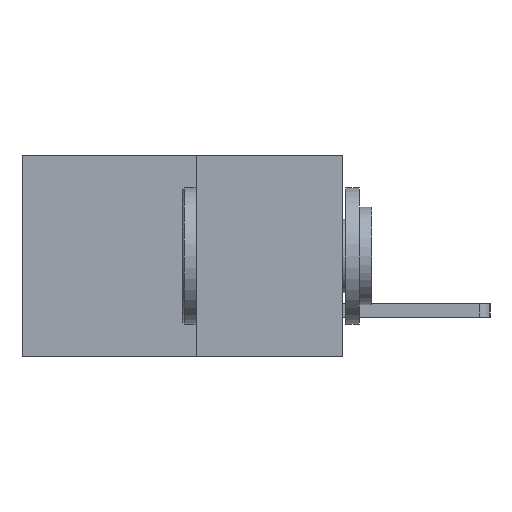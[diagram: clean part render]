
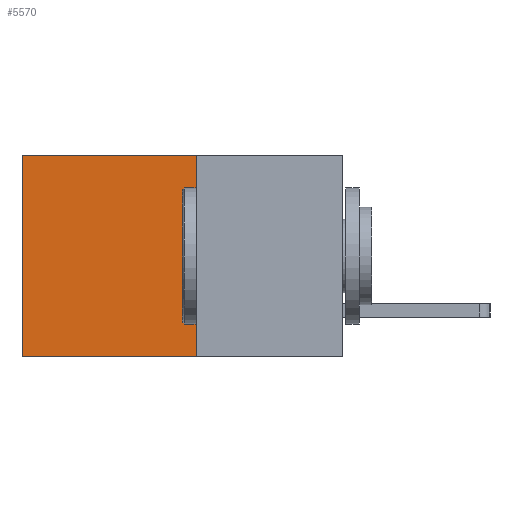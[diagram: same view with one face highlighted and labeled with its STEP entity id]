
A CAD part, left-side view. The second image highlights one B-rep face of the part: STEP entity #5570.
In plain terms, the highlighted planar face has unit normal (-1, 0, 0).
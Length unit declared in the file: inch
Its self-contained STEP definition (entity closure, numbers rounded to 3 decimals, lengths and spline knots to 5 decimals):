
#22 = ORIENTED_EDGE ( 'NONE', *, *, #4713, .T. ) ;
#277 = EDGE_CURVE ( 'NONE', #1090, #2501, #8124, .T. ) ;
#381 = DIRECTION ( 'NONE',  ( 0., 0., -1. ) ) ;
#455 = VECTOR ( 'NONE', #1101, 39.37008 ) ;
#534 = DIRECTION ( 'NONE',  ( 1., 0., 0. ) ) ;
#548 = CARTESIAN_POINT ( 'NONE',  ( 0.277, 0.27, -0.37 ) ) ;
#688 = PLANE ( 'NONE',  #2563 ) ;
#1090 = VERTEX_POINT ( 'NONE', #5606 ) ;
#1101 = DIRECTION ( 'NONE',  ( 0., 0., -1. ) ) ;
#1481 = CARTESIAN_POINT ( 'NONE',  ( 0.277, 0.27, -0.37 ) ) ;
#1509 = EDGE_LOOP ( 'NONE', ( #22, #2766, #8586, #7728 ) ) ;
#2123 = VERTEX_POINT ( 'NONE', #7478 ) ;
#2501 = VERTEX_POINT ( 'NONE', #4566 ) ;
#2563 = AXIS2_PLACEMENT_3D ( 'NONE', #548, #534, #381 ) ;
#2648 = VECTOR ( 'NONE', #8681, 39.37008 ) ;
#2766 = ORIENTED_EDGE ( 'NONE', *, *, #277, .F. ) ;
#4310 = LINE ( 'NONE', #1481, #455 ) ;
#4478 = CARTESIAN_POINT ( 'NONE',  ( 0.277, 0.27, 0. ) ) ;
#4566 = CARTESIAN_POINT ( 'NONE',  ( 0.277, 0.59, -0.37 ) ) ;
#4713 = EDGE_CURVE ( 'NONE', #2123, #2501, #5954, .T. ) ;
#5328 = EDGE_CURVE ( 'NONE', #7830, #2123, #7575, .T. ) ;
#5570 = ADVANCED_FACE ( 'NONE', ( #7466 ), #688, .F. ) ;
#5606 = CARTESIAN_POINT ( 'NONE',  ( 0.277, 0.27, -0.37 ) ) ;
#5683 = VECTOR ( 'NONE', #8881, 39.37008 ) ;
#5719 = VECTOR ( 'NONE', #7019, 39.37008 ) ;
#5932 = CARTESIAN_POINT ( 'NONE',  ( 0.277, 0.27, -0.37 ) ) ;
#5954 = LINE ( 'NONE', #7749, #5719 ) ;
#6415 = EDGE_CURVE ( 'NONE', #7830, #1090, #4310, .T. ) ;
#7019 = DIRECTION ( 'NONE',  ( 0., 0., -1. ) ) ;
#7466 = FACE_OUTER_BOUND ( 'NONE', #1509, .T. ) ;
#7478 = CARTESIAN_POINT ( 'NONE',  ( 0.277, 0.59, 0. ) ) ;
#7575 = LINE ( 'NONE', #8238, #5683 ) ;
#7728 = ORIENTED_EDGE ( 'NONE', *, *, #5328, .T. ) ;
#7749 = CARTESIAN_POINT ( 'NONE',  ( 0.277, 0.59, -0.37 ) ) ;
#7830 = VERTEX_POINT ( 'NONE', #4478 ) ;
#8124 = LINE ( 'NONE', #5932, #2648 ) ;
#8238 = CARTESIAN_POINT ( 'NONE',  ( 0.277, 0.27, 0. ) ) ;
#8586 = ORIENTED_EDGE ( 'NONE', *, *, #6415, .F. ) ;
#8681 = DIRECTION ( 'NONE',  ( 0., 1., 0. ) ) ;
#8881 = DIRECTION ( 'NONE',  ( 0., 1., 0. ) ) ;
